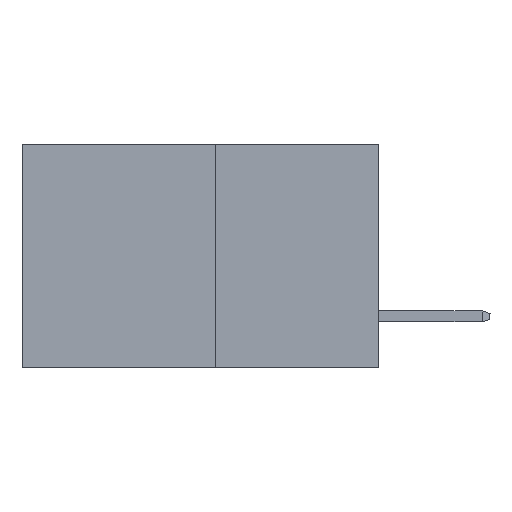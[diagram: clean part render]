
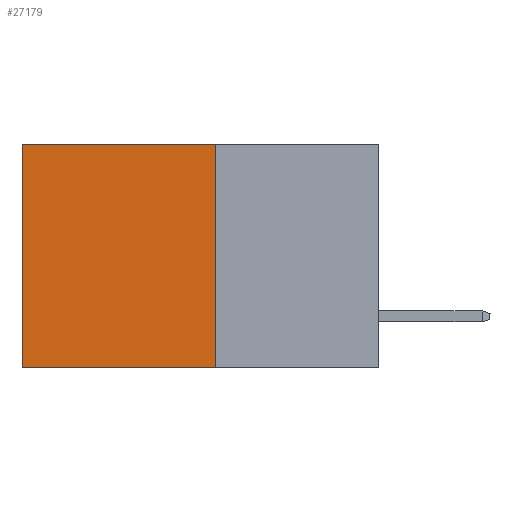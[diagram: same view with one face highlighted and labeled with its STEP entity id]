
A CAD part, left-side view. The second image highlights one B-rep face of the part: STEP entity #27179.
In plain terms, the highlighted planar face has unit normal (-1, 0, 0).
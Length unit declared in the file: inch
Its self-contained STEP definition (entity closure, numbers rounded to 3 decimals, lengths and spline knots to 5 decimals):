
#492 = CARTESIAN_POINT ( 'NONE',  ( 0.277, 0.27, -0.37 ) ) ;
#650 = DIRECTION ( 'NONE',  ( 0., 1., 0. ) ) ;
#2060 = VECTOR ( 'NONE', #4166, 39.37008 ) ;
#2419 = ORIENTED_EDGE ( 'NONE', *, *, #3704, .F. ) ;
#2793 = EDGE_CURVE ( 'NONE', #18132, #15506, #9689, .T. ) ;
#3465 = CARTESIAN_POINT ( 'NONE',  ( 0.277, 0.27, 0. ) ) ;
#3669 = ORIENTED_EDGE ( 'NONE', *, *, #2793, .T. ) ;
#3704 = EDGE_CURVE ( 'NONE', #26591, #25226, #12853, .T. ) ;
#4166 = DIRECTION ( 'NONE',  ( 0., 1., 0. ) ) ;
#6036 = VECTOR ( 'NONE', #650, 39.37008 ) ;
#6512 = EDGE_CURVE ( 'NONE', #18132, #26591, #28795, .T. ) ;
#8020 = VECTOR ( 'NONE', #28960, 39.37008 ) ;
#9255 = DIRECTION ( 'NONE',  ( 0., 0., -1. ) ) ;
#9686 = FACE_OUTER_BOUND ( 'NONE', #12425, .T. ) ;
#9689 = LINE ( 'NONE', #3465, #2060 ) ;
#10116 = EDGE_CURVE ( 'NONE', #15506, #25226, #22508, .T. ) ;
#10175 = CARTESIAN_POINT ( 'NONE',  ( 0.277, 0.27, -0.37 ) ) ;
#10598 = AXIS2_PLACEMENT_3D ( 'NONE', #10175, #28201, #12716 ) ;
#11448 = ORIENTED_EDGE ( 'NONE', *, *, #10116, .T. ) ;
#11950 = CARTESIAN_POINT ( 'NONE',  ( 0.277, 0.27, 0. ) ) ;
#12211 = CARTESIAN_POINT ( 'NONE',  ( 0.277, 0.27, -0.37 ) ) ;
#12425 = EDGE_LOOP ( 'NONE', ( #11448, #2419, #28245, #3669 ) ) ;
#12716 = DIRECTION ( 'NONE',  ( 0., 0., -1. ) ) ;
#12853 = LINE ( 'NONE', #492, #6036 ) ;
#12942 = CARTESIAN_POINT ( 'NONE',  ( 0.277, 0.59, -0.37 ) ) ;
#15506 = VERTEX_POINT ( 'NONE', #30925 ) ;
#18132 = VERTEX_POINT ( 'NONE', #11950 ) ;
#18177 = CARTESIAN_POINT ( 'NONE',  ( 0.277, 0.27, -0.37 ) ) ;
#21908 = VECTOR ( 'NONE', #9255, 39.37008 ) ;
#22508 = LINE ( 'NONE', #12942, #8020 ) ;
#25226 = VERTEX_POINT ( 'NONE', #27185 ) ;
#26591 = VERTEX_POINT ( 'NONE', #18177 ) ;
#27179 = ADVANCED_FACE ( 'NONE', ( #9686 ), #33350, .F. ) ;
#27185 = CARTESIAN_POINT ( 'NONE',  ( 0.277, 0.59, -0.37 ) ) ;
#28201 = DIRECTION ( 'NONE',  ( 1., 0., 0. ) ) ;
#28245 = ORIENTED_EDGE ( 'NONE', *, *, #6512, .F. ) ;
#28795 = LINE ( 'NONE', #12211, #21908 ) ;
#28960 = DIRECTION ( 'NONE',  ( 0., 0., -1. ) ) ;
#30925 = CARTESIAN_POINT ( 'NONE',  ( 0.277, 0.59, 0. ) ) ;
#33350 = PLANE ( 'NONE',  #10598 ) ;
